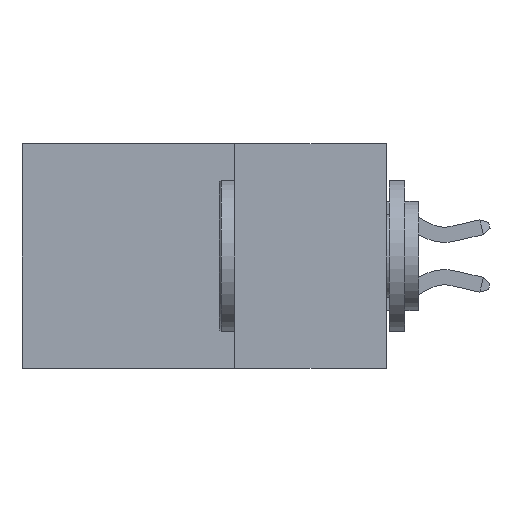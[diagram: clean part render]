
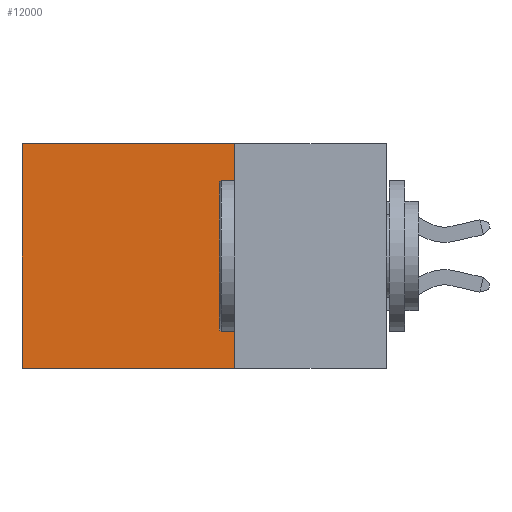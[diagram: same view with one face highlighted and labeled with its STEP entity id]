
A CAD part, left-side view. The second image highlights one B-rep face of the part: STEP entity #12000.
In plain terms, the highlighted planar face has unit normal (-1, 0, 0).
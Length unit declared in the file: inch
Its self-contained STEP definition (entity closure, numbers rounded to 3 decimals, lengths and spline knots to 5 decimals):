
#99 = CARTESIAN_POINT ( 'NONE',  ( 0.2615, 0.25, 0. ) ) ;
#156 = DIRECTION ( 'NONE',  ( 0., 0., -1. ) ) ;
#2312 = DIRECTION ( 'NONE',  ( 0., 1., 0. ) ) ;
#2603 = CARTESIAN_POINT ( 'NONE',  ( 0.2615, 0.25, -0.37 ) ) ;
#2843 = VERTEX_POINT ( 'NONE', #2603 ) ;
#3150 = VECTOR ( 'NONE', #5190, 39.37008 ) ;
#3926 = ORIENTED_EDGE ( 'NONE', *, *, #12674, .F. ) ;
#3936 = EDGE_CURVE ( 'NONE', #11433, #13405, #5391, .T. ) ;
#4335 = EDGE_LOOP ( 'NONE', ( #11910, #13322, #3926, #10127 ) ) ;
#4368 = LINE ( 'NONE', #5274, #9388 ) ;
#4806 = EDGE_CURVE ( 'NONE', #2843, #13405, #4368, .T. ) ;
#5124 = DIRECTION ( 'NONE',  ( 0., 0., -1. ) ) ;
#5190 = DIRECTION ( 'NONE',  ( 0., 1., 0. ) ) ;
#5274 = CARTESIAN_POINT ( 'NONE',  ( 0.2615, 0.25, -0.37 ) ) ;
#5391 = LINE ( 'NONE', #7346, #11778 ) ;
#6667 = VERTEX_POINT ( 'NONE', #12741 ) ;
#6905 = CARTESIAN_POINT ( 'NONE',  ( 0.2615, 0.6, 0. ) ) ;
#7340 = DIRECTION ( 'NONE',  ( 0., 0., -1. ) ) ;
#7346 = CARTESIAN_POINT ( 'NONE',  ( 0.2615, 0.6, -0.37 ) ) ;
#8042 = CARTESIAN_POINT ( 'NONE',  ( 0.2615, 0.25, -0.37 ) ) ;
#8422 = VECTOR ( 'NONE', #7340, 39.37008 ) ;
#9147 = FACE_OUTER_BOUND ( 'NONE', #4335, .T. ) ;
#9388 = VECTOR ( 'NONE', #2312, 39.37008 ) ;
#9485 = LINE ( 'NONE', #99, #3150 ) ;
#10127 = ORIENTED_EDGE ( 'NONE', *, *, #10879, .T. ) ;
#10563 = CARTESIAN_POINT ( 'NONE',  ( 0.2615, 0.25, -0.37 ) ) ;
#10879 = EDGE_CURVE ( 'NONE', #6667, #11433, #9485, .T. ) ;
#11433 = VERTEX_POINT ( 'NONE', #6905 ) ;
#11680 = AXIS2_PLACEMENT_3D ( 'NONE', #8042, #13307, #5124 ) ;
#11726 = LINE ( 'NONE', #10563, #8422 ) ;
#11778 = VECTOR ( 'NONE', #156, 39.37008 ) ;
#11910 = ORIENTED_EDGE ( 'NONE', *, *, #3936, .T. ) ;
#12000 = ADVANCED_FACE ( 'NONE', ( #9147 ), #13242, .F. ) ;
#12674 = EDGE_CURVE ( 'NONE', #6667, #2843, #11726, .T. ) ;
#12741 = CARTESIAN_POINT ( 'NONE',  ( 0.2615, 0.25, 0. ) ) ;
#13180 = CARTESIAN_POINT ( 'NONE',  ( 0.2615, 0.6, -0.37 ) ) ;
#13242 = PLANE ( 'NONE',  #11680 ) ;
#13307 = DIRECTION ( 'NONE',  ( 1., 0., 0. ) ) ;
#13322 = ORIENTED_EDGE ( 'NONE', *, *, #4806, .F. ) ;
#13405 = VERTEX_POINT ( 'NONE', #13180 ) ;
